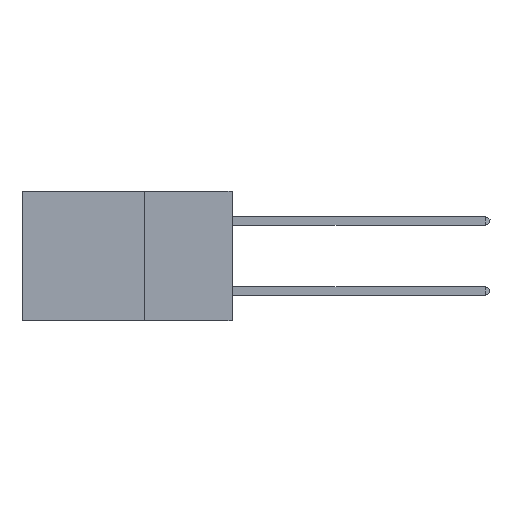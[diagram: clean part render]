
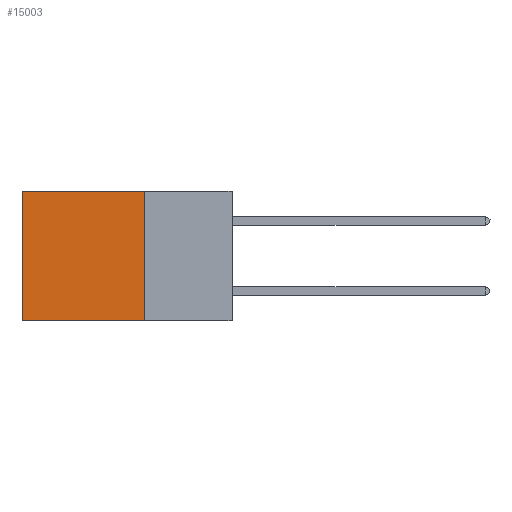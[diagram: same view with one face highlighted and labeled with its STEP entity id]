
A CAD part, left-side view. The second image highlights one B-rep face of the part: STEP entity #15003.
In plain terms, the highlighted planar face has unit normal (-1, 0, 0).
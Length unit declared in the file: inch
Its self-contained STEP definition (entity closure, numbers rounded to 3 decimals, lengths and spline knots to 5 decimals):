
#1252 = DIRECTION ( 'NONE',  ( 0., 0., -1. ) ) ;
#3819 = DIRECTION ( 'NONE',  ( 0., 0., -1. ) ) ;
#6093 = VERTEX_POINT ( 'NONE', #23182 ) ;
#7169 = VERTEX_POINT ( 'NONE', #45083 ) ;
#9371 = CARTESIAN_POINT ( 'NONE',  ( 0.2875, 0.6, 0. ) ) ;
#12001 = EDGE_LOOP ( 'NONE', ( #32715, #32292, #30327, #44834 ) ) ;
#13030 = DIRECTION ( 'NONE',  ( 0., 0., -1. ) ) ;
#13341 = DIRECTION ( 'NONE',  ( 0., 1., 0. ) ) ;
#15003 = ADVANCED_FACE ( 'NONE', ( #26268 ), #18109, .F. ) ;
#15420 = EDGE_CURVE ( 'NONE', #6093, #31055, #33157, .T. ) ;
#15703 = CARTESIAN_POINT ( 'NONE',  ( 0.2875, 0.25, 0. ) ) ;
#18109 = PLANE ( 'NONE',  #21564 ) ;
#18310 = CARTESIAN_POINT ( 'NONE',  ( 0.2875, 0.6, -0.37 ) ) ;
#20660 = CARTESIAN_POINT ( 'NONE',  ( 0.2875, 0.25, 0. ) ) ;
#21564 = AXIS2_PLACEMENT_3D ( 'NONE', #21669, #25202, #3819 ) ;
#21669 = CARTESIAN_POINT ( 'NONE',  ( 0.2875, 0.25, 0. ) ) ;
#23182 = CARTESIAN_POINT ( 'NONE',  ( 0.2875, 0.25, -0.37 ) ) ;
#24885 = EDGE_CURVE ( 'NONE', #7169, #6093, #37086, .T. ) ;
#25202 = DIRECTION ( 'NONE',  ( 1., 0., 0. ) ) ;
#25914 = VERTEX_POINT ( 'NONE', #44761 ) ;
#26240 = LINE ( 'NONE', #9371, #35282 ) ;
#26268 = FACE_OUTER_BOUND ( 'NONE', #12001, .T. ) ;
#30327 = ORIENTED_EDGE ( 'NONE', *, *, #24885, .F. ) ;
#31055 = VERTEX_POINT ( 'NONE', #18310 ) ;
#32292 = ORIENTED_EDGE ( 'NONE', *, *, #15420, .F. ) ;
#32715 = ORIENTED_EDGE ( 'NONE', *, *, #40711, .T. ) ;
#33157 = LINE ( 'NONE', #37476, #41040 ) ;
#35282 = VECTOR ( 'NONE', #13030, 39.37008 ) ;
#37086 = LINE ( 'NONE', #15703, #44896 ) ;
#37476 = CARTESIAN_POINT ( 'NONE',  ( 0.2875, 0.25, -0.37 ) ) ;
#40711 = EDGE_CURVE ( 'NONE', #25914, #31055, #26240, .T. ) ;
#41040 = VECTOR ( 'NONE', #13341, 39.37008 ) ;
#41390 = EDGE_CURVE ( 'NONE', #7169, #25914, #42093, .T. ) ;
#42093 = LINE ( 'NONE', #20660, #44191 ) ;
#44191 = VECTOR ( 'NONE', #44437, 39.37008 ) ;
#44437 = DIRECTION ( 'NONE',  ( 0., 1., 0. ) ) ;
#44761 = CARTESIAN_POINT ( 'NONE',  ( 0.2875, 0.6, 0. ) ) ;
#44834 = ORIENTED_EDGE ( 'NONE', *, *, #41390, .T. ) ;
#44896 = VECTOR ( 'NONE', #1252, 39.37008 ) ;
#45083 = CARTESIAN_POINT ( 'NONE',  ( 0.2875, 0.25, 0. ) ) ;
